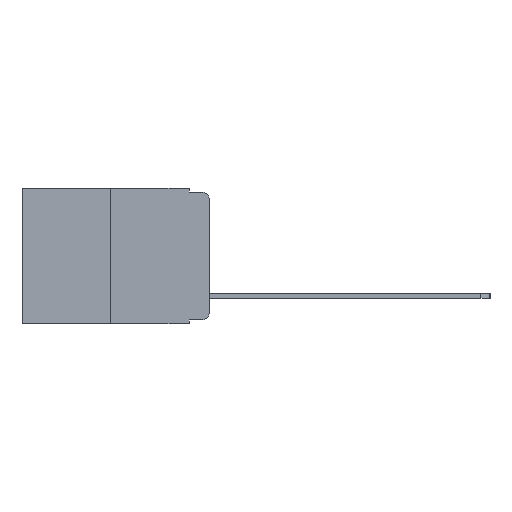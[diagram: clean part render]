
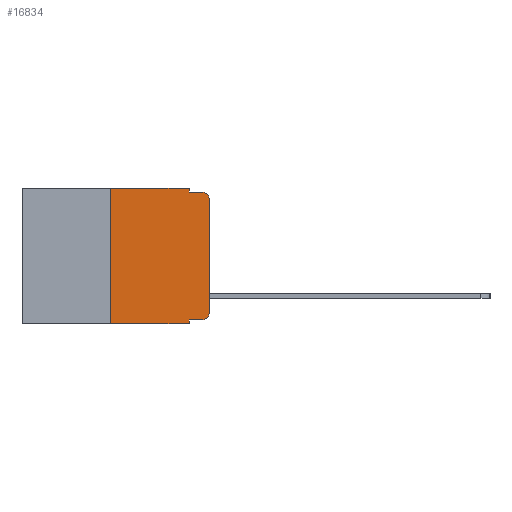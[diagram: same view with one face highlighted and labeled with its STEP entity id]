
A CAD part, left-side view. The second image highlights one B-rep face of the part: STEP entity #16834.
In plain terms, the highlighted planar face has unit normal (-1, 0, 0).
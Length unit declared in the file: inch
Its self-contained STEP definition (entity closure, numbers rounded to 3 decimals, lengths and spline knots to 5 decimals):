
#213 = LINE ( 'NONE', #4748, #15808 ) ;
#246 = VERTEX_POINT ( 'NONE', #11001 ) ;
#342 = CARTESIAN_POINT ( 'NONE',  ( 0., 0.051, 0. ) ) ;
#515 = CARTESIAN_POINT ( 'NONE',  ( 0., 0.051, -0.333 ) ) ;
#690 = ORIENTED_EDGE ( 'NONE', *, *, #11046, .F. ) ;
#1016 = CARTESIAN_POINT ( 'NONE',  ( 0., 0.02, -0.01 ) ) ;
#1235 = VERTEX_POINT ( 'NONE', #1016 ) ;
#1249 = VECTOR ( 'NONE', #6734, 39.37008 ) ;
#1723 = VECTOR ( 'NONE', #15687, 39.37008 ) ;
#1844 = FACE_OUTER_BOUND ( 'NONE', #15505, .T. ) ;
#2132 = CARTESIAN_POINT ( 'NONE',  ( 0., 0.051, 0. ) ) ;
#2707 = VERTEX_POINT ( 'NONE', #5762 ) ;
#2709 = AXIS2_PLACEMENT_3D ( 'NONE', #3536, #8195, #18330 ) ;
#2835 = AXIS2_PLACEMENT_3D ( 'NONE', #13055, #4053, #14515 ) ;
#2977 = CARTESIAN_POINT ( 'NONE',  ( 0., 0.051, -0.01 ) ) ;
#3344 = VERTEX_POINT ( 'NONE', #17080 ) ;
#3536 = CARTESIAN_POINT ( 'NONE',  ( 0., 0.473, 0. ) ) ;
#3672 = VECTOR ( 'NONE', #8728, 39.37008 ) ;
#4053 = DIRECTION ( 'NONE',  ( -1., 0., 0. ) ) ;
#4066 = CIRCLE ( 'NONE', #9889, 0.02 ) ;
#4594 = EDGE_CURVE ( 'NONE', #10269, #10885, #5826, .T. ) ;
#4748 = CARTESIAN_POINT ( 'NONE',  ( 0., 0.25, 0. ) ) ;
#5707 = VECTOR ( 'NONE', #8414, 39.37008 ) ;
#5762 = CARTESIAN_POINT ( 'NONE',  ( 0., 0., -0.313 ) ) ;
#5826 = LINE ( 'NONE', #7853, #13741 ) ;
#5886 = DIRECTION ( 'NONE',  ( 0., -1., 0. ) ) ;
#6300 = DIRECTION ( 'NONE',  ( -1., 0., 0. ) ) ;
#6653 = PLANE ( 'NONE',  #2709 ) ;
#6734 = DIRECTION ( 'NONE',  ( 0., -1., 0. ) ) ;
#6876 = CARTESIAN_POINT ( 'NONE',  ( 0., 0., 0. ) ) ;
#7237 = EDGE_CURVE ( 'NONE', #246, #2707, #4066, .T. ) ;
#7290 = VECTOR ( 'NONE', #15768, 39.37008 ) ;
#7853 = CARTESIAN_POINT ( 'NONE',  ( 0., 0.473, 0. ) ) ;
#7865 = CARTESIAN_POINT ( 'NONE',  ( 0., 0.051, -0.333 ) ) ;
#8195 = DIRECTION ( 'NONE',  ( 1., 0., 0. ) ) ;
#8414 = DIRECTION ( 'NONE',  ( 0., 0., -1. ) ) ;
#8511 = CARTESIAN_POINT ( 'NONE',  ( 0., 0.051, -0.01 ) ) ;
#8638 = ORIENTED_EDGE ( 'NONE', *, *, #7237, .T. ) ;
#8728 = DIRECTION ( 'NONE',  ( 0., 0., -1. ) ) ;
#9512 = LINE ( 'NONE', #14754, #17184 ) ;
#9762 = EDGE_CURVE ( 'NONE', #16797, #246, #17152, .T. ) ;
#9773 = LINE ( 'NONE', #2132, #5707 ) ;
#9786 = EDGE_CURVE ( 'NONE', #2707, #3344, #16728, .T. ) ;
#9889 = AXIS2_PLACEMENT_3D ( 'NONE', #15148, #6300, #16593 ) ;
#10088 = ORIENTED_EDGE ( 'NONE', *, *, #9786, .T. ) ;
#10269 = VERTEX_POINT ( 'NONE', #15349 ) ;
#10550 = EDGE_CURVE ( 'NONE', #3344, #1235, #15574, .T. ) ;
#10579 = EDGE_CURVE ( 'NONE', #10885, #14850, #15127, .T. ) ;
#10829 = ORIENTED_EDGE ( 'NONE', *, *, #10579, .F. ) ;
#10885 = VERTEX_POINT ( 'NONE', #342 ) ;
#11001 = CARTESIAN_POINT ( 'NONE',  ( 0., 0.02, -0.333 ) ) ;
#11046 = EDGE_CURVE ( 'NONE', #14850, #1235, #11262, .T. ) ;
#11149 = ORIENTED_EDGE ( 'NONE', *, *, #9762, .T. ) ;
#11262 = LINE ( 'NONE', #8511, #7290 ) ;
#11637 = VERTEX_POINT ( 'NONE', #18295 ) ;
#12013 = ORIENTED_EDGE ( 'NONE', *, *, #18311, .F. ) ;
#12372 = VERTEX_POINT ( 'NONE', #13837 ) ;
#13055 = CARTESIAN_POINT ( 'NONE',  ( 0., 0.02, -0.03 ) ) ;
#13741 = VECTOR ( 'NONE', #16595, 39.37008 ) ;
#13816 = ORIENTED_EDGE ( 'NONE', *, *, #14955, .F. ) ;
#13837 = CARTESIAN_POINT ( 'NONE',  ( 0., 0.051, -0.343 ) ) ;
#14515 = DIRECTION ( 'NONE',  ( 0., 0., -1. ) ) ;
#14754 = CARTESIAN_POINT ( 'NONE',  ( 0., 0.473, -0.343 ) ) ;
#14850 = VERTEX_POINT ( 'NONE', #2977 ) ;
#14870 = ORIENTED_EDGE ( 'NONE', *, *, #10550, .T. ) ;
#14955 = EDGE_CURVE ( 'NONE', #11637, #10269, #213, .T. ) ;
#15127 = LINE ( 'NONE', #18807, #3672 ) ;
#15148 = CARTESIAN_POINT ( 'NONE',  ( 0., 0.02, -0.313 ) ) ;
#15349 = CARTESIAN_POINT ( 'NONE',  ( 0., 0.25, 0. ) ) ;
#15505 = EDGE_LOOP ( 'NONE', ( #10088, #14870, #690, #10829, #16481, #13816, #16943, #12013, #11149, #8638 ) ) ;
#15574 = CIRCLE ( 'NONE', #2835, 0.02 ) ;
#15687 = DIRECTION ( 'NONE',  ( 0., 0., 1. ) ) ;
#15768 = DIRECTION ( 'NONE',  ( 0., -1., 0. ) ) ;
#15808 = VECTOR ( 'NONE', #18020, 39.37008 ) ;
#16481 = ORIENTED_EDGE ( 'NONE', *, *, #4594, .F. ) ;
#16593 = DIRECTION ( 'NONE',  ( 0., 0., -1. ) ) ;
#16595 = DIRECTION ( 'NONE',  ( 0., -1., 0. ) ) ;
#16728 = LINE ( 'NONE', #6876, #1723 ) ;
#16797 = VERTEX_POINT ( 'NONE', #7865 ) ;
#16834 = ADVANCED_FACE ( 'NONE', ( #1844 ), #6653, .F. ) ;
#16943 = ORIENTED_EDGE ( 'NONE', *, *, #19017, .T. ) ;
#17080 = CARTESIAN_POINT ( 'NONE',  ( 0., 0., -0.03 ) ) ;
#17152 = LINE ( 'NONE', #515, #1249 ) ;
#17184 = VECTOR ( 'NONE', #5886, 39.37008 ) ;
#18020 = DIRECTION ( 'NONE',  ( 0., 0., 1. ) ) ;
#18295 = CARTESIAN_POINT ( 'NONE',  ( 0., 0.25, -0.343 ) ) ;
#18311 = EDGE_CURVE ( 'NONE', #16797, #12372, #9773, .T. ) ;
#18330 = DIRECTION ( 'NONE',  ( 0., 0., -1. ) ) ;
#18807 = CARTESIAN_POINT ( 'NONE',  ( 0., 0.051, 0. ) ) ;
#19017 = EDGE_CURVE ( 'NONE', #11637, #12372, #9512, .T. ) ;
